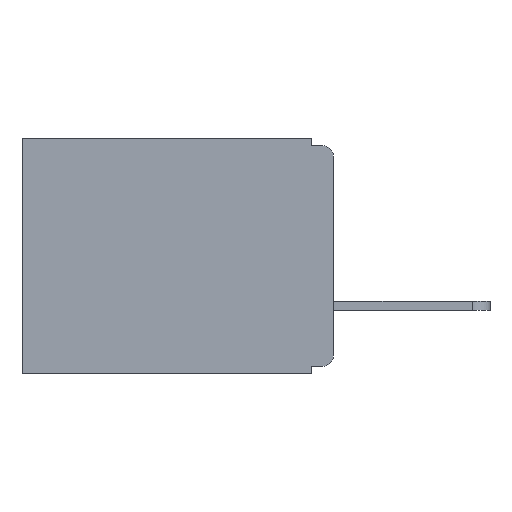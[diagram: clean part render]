
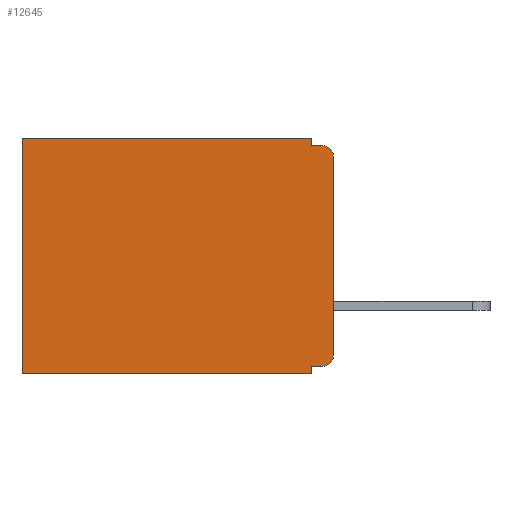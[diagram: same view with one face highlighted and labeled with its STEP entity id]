
A CAD part, left-side view. The second image highlights one B-rep face of the part: STEP entity #12645.
In plain terms, the highlighted planar face has unit normal (-1, 0, 0).
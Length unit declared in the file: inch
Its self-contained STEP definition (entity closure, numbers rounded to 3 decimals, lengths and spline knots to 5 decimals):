
#139 = DIRECTION ( 'NONE',  ( 0., 0., -1. ) ) ;
#268 = CARTESIAN_POINT ( 'NONE',  ( 0.3, 0., 0. ) ) ;
#292 = DIRECTION ( 'NONE',  ( 1., 0., 0. ) ) ;
#300 = EDGE_CURVE ( 'NONE', #3900, #12633, #8066, .T. ) ;
#493 = VERTEX_POINT ( 'NONE', #9127 ) ;
#537 = VERTEX_POINT ( 'NONE', #3351 ) ;
#716 = DIRECTION ( 'NONE',  ( 0., 0., -1. ) ) ;
#796 = ORIENTED_EDGE ( 'NONE', *, *, #300, .T. ) ;
#1519 = EDGE_CURVE ( 'NONE', #11154, #6484, #10776, .T. ) ;
#1759 = LINE ( 'NONE', #5209, #10435 ) ;
#1983 = ORIENTED_EDGE ( 'NONE', *, *, #4203, .F. ) ;
#2074 = AXIS2_PLACEMENT_3D ( 'NONE', #10117, #6224, #9021 ) ;
#2085 = ORIENTED_EDGE ( 'NONE', *, *, #1519, .T. ) ;
#2141 = VERTEX_POINT ( 'NONE', #9541 ) ;
#2218 = PLANE ( 'NONE',  #5668 ) ;
#2233 = DIRECTION ( 'NONE',  ( 0., 1., 0. ) ) ;
#2265 = CARTESIAN_POINT ( 'NONE',  ( 0.3, 0.437, 0. ) ) ;
#2382 = EDGE_CURVE ( 'NONE', #493, #2141, #1759, .T. ) ;
#2465 = ORIENTED_EDGE ( 'NONE', *, *, #2382, .F. ) ;
#2833 = VERTEX_POINT ( 'NONE', #6745 ) ;
#3004 = CARTESIAN_POINT ( 'NONE',  ( 0.3, 0.437, -0.33 ) ) ;
#3133 = DIRECTION ( 'NONE',  ( 0., -1., 0. ) ) ;
#3192 = CARTESIAN_POINT ( 'NONE',  ( 0.3, 0.031, 0. ) ) ;
#3237 = CIRCLE ( 'NONE', #2074, 0.015 ) ;
#3351 = CARTESIAN_POINT ( 'NONE',  ( 0.3, 0.031, -0.32 ) ) ;
#3617 = DIRECTION ( 'NONE',  ( 0., 0., -1. ) ) ;
#3783 = FACE_OUTER_BOUND ( 'NONE', #9348, .T. ) ;
#3802 = ORIENTED_EDGE ( 'NONE', *, *, #7236, .F. ) ;
#3882 = VECTOR ( 'NONE', #8559, 39.37008 ) ;
#3900 = VERTEX_POINT ( 'NONE', #12428 ) ;
#4203 = EDGE_CURVE ( 'NONE', #537, #6222, #10742, .T. ) ;
#4373 = CARTESIAN_POINT ( 'NONE',  ( 0.3, 0.031, -0.33 ) ) ;
#4462 = VECTOR ( 'NONE', #10842, 39.37008 ) ;
#4599 = EDGE_CURVE ( 'NONE', #5467, #6484, #11948, .T. ) ;
#4703 = EDGE_CURVE ( 'NONE', #11154, #537, #6451, .T. ) ;
#4780 = VECTOR ( 'NONE', #716, 39.37008 ) ;
#4959 = DIRECTION ( 'NONE',  ( 0., 0., -1. ) ) ;
#5132 = ORIENTED_EDGE ( 'NONE', *, *, #6084, .T. ) ;
#5183 = LINE ( 'NONE', #3004, #5944 ) ;
#5208 = CARTESIAN_POINT ( 'NONE',  ( 0.3, 0., -0.33 ) ) ;
#5209 = CARTESIAN_POINT ( 'NONE',  ( 0.3, 0., -0.01 ) ) ;
#5313 = DIRECTION ( 'NONE',  ( 0., 0., -1. ) ) ;
#5467 = VERTEX_POINT ( 'NONE', #6134 ) ;
#5668 = AXIS2_PLACEMENT_3D ( 'NONE', #9052, #292, #5313 ) ;
#5944 = VECTOR ( 'NONE', #139, 39.37008 ) ;
#6084 = EDGE_CURVE ( 'NONE', #5467, #2141, #3237, .T. ) ;
#6134 = CARTESIAN_POINT ( 'NONE',  ( 0.3, 0., -0.025 ) ) ;
#6222 = VERTEX_POINT ( 'NONE', #4373 ) ;
#6224 = DIRECTION ( 'NONE',  ( -1., 0., 0. ) ) ;
#6400 = CARTESIAN_POINT ( 'NONE',  ( 0.3, 0., -0.33 ) ) ;
#6451 = LINE ( 'NONE', #7584, #3882 ) ;
#6484 = VERTEX_POINT ( 'NONE', #11389 ) ;
#6745 = CARTESIAN_POINT ( 'NONE',  ( 0.3, 0.437, -0.33 ) ) ;
#7151 = EDGE_CURVE ( 'NONE', #12633, #2833, #5183, .T. ) ;
#7236 = EDGE_CURVE ( 'NONE', #6222, #2833, #10193, .T. ) ;
#7515 = DIRECTION ( 'NONE',  ( -1., 0., 0. ) ) ;
#7584 = CARTESIAN_POINT ( 'NONE',  ( 0.3, 0., -0.32 ) ) ;
#7904 = ORIENTED_EDGE ( 'NONE', *, *, #4599, .F. ) ;
#8066 = LINE ( 'NONE', #268, #8365 ) ;
#8365 = VECTOR ( 'NONE', #10010, 39.37008 ) ;
#8559 = DIRECTION ( 'NONE',  ( 0., 1., 0. ) ) ;
#8708 = CARTESIAN_POINT ( 'NONE',  ( 0.3, 0.015, -0.32 ) ) ;
#8804 = EDGE_CURVE ( 'NONE', #3900, #493, #9638, .T. ) ;
#8973 = VECTOR ( 'NONE', #2233, 39.37008 ) ;
#9021 = DIRECTION ( 'NONE',  ( 0., 0., -1. ) ) ;
#9052 = CARTESIAN_POINT ( 'NONE',  ( 0.3, 0., -0.33 ) ) ;
#9127 = CARTESIAN_POINT ( 'NONE',  ( 0.3, 0.031, -0.01 ) ) ;
#9348 = EDGE_LOOP ( 'NONE', ( #7904, #5132, #2465, #11097, #796, #9414, #3802, #1983, #12006, #2085 ) ) ;
#9414 = ORIENTED_EDGE ( 'NONE', *, *, #7151, .T. ) ;
#9541 = CARTESIAN_POINT ( 'NONE',  ( 0.3, 0.015, -0.01 ) ) ;
#9638 = LINE ( 'NONE', #3192, #4462 ) ;
#10010 = DIRECTION ( 'NONE',  ( 0., 1., 0. ) ) ;
#10117 = CARTESIAN_POINT ( 'NONE',  ( 0.3, 0.015, -0.025 ) ) ;
#10193 = LINE ( 'NONE', #5208, #8973 ) ;
#10435 = VECTOR ( 'NONE', #3133, 39.37008 ) ;
#10669 = CARTESIAN_POINT ( 'NONE',  ( 0.3, 0.031, -0.33 ) ) ;
#10742 = LINE ( 'NONE', #10669, #12578 ) ;
#10776 = CIRCLE ( 'NONE', #12079, 0.015 ) ;
#10842 = DIRECTION ( 'NONE',  ( 0., 0., -1. ) ) ;
#11097 = ORIENTED_EDGE ( 'NONE', *, *, #8804, .F. ) ;
#11154 = VERTEX_POINT ( 'NONE', #8708 ) ;
#11389 = CARTESIAN_POINT ( 'NONE',  ( 0.3, 0., -0.305 ) ) ;
#11573 = CARTESIAN_POINT ( 'NONE',  ( 0.3, 0.015, -0.305 ) ) ;
#11948 = LINE ( 'NONE', #6400, #4780 ) ;
#12006 = ORIENTED_EDGE ( 'NONE', *, *, #4703, .F. ) ;
#12079 = AXIS2_PLACEMENT_3D ( 'NONE', #11573, #7515, #3617 ) ;
#12428 = CARTESIAN_POINT ( 'NONE',  ( 0.3, 0.031, 0. ) ) ;
#12578 = VECTOR ( 'NONE', #4959, 39.37008 ) ;
#12633 = VERTEX_POINT ( 'NONE', #2265 ) ;
#12645 = ADVANCED_FACE ( 'NONE', ( #3783 ), #2218, .F. ) ;
